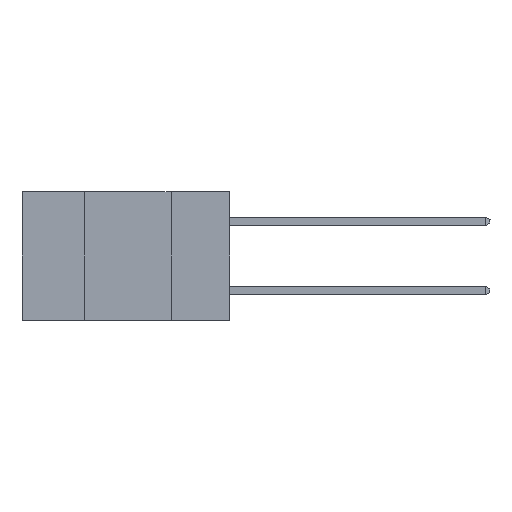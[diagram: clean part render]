
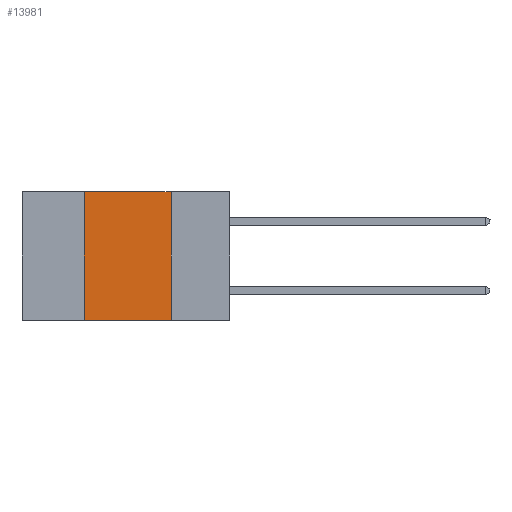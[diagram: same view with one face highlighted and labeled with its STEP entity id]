
A CAD part, left-side view. The second image highlights one B-rep face of the part: STEP entity #13981.
In plain terms, the highlighted planar face has unit normal (-1, 0, 0).
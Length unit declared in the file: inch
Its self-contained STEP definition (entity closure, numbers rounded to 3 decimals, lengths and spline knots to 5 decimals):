
#1023 = DIRECTION ( 'NONE',  ( 0., 0., 1. ) ) ;
#4961 = CARTESIAN_POINT ( 'NONE',  ( 0., 0.6, 0. ) ) ;
#5882 = LINE ( 'NONE', #26419, #10526 ) ;
#6007 = VECTOR ( 'NONE', #11880, 39.37008 ) ;
#7266 = DIRECTION ( 'NONE',  ( 0., 0., -1. ) ) ;
#7350 = FACE_OUTER_BOUND ( 'NONE', #15624, .T. ) ;
#8028 = CARTESIAN_POINT ( 'NONE',  ( 0., 0.42, 0. ) ) ;
#8097 = VECTOR ( 'NONE', #1023, 39.37008 ) ;
#8830 = CARTESIAN_POINT ( 'NONE',  ( 0., 0.42, 0. ) ) ;
#9440 = ORIENTED_EDGE ( 'NONE', *, *, #19440, .F. ) ;
#9848 = PLANE ( 'NONE',  #13588 ) ;
#10526 = VECTOR ( 'NONE', #26039, 39.37008 ) ;
#11048 = LINE ( 'NONE', #26996, #16787 ) ;
#11230 = DIRECTION ( 'NONE',  ( 0., -1., 0. ) ) ;
#11699 = ORIENTED_EDGE ( 'NONE', *, *, #18693, .F. ) ;
#11793 = CARTESIAN_POINT ( 'NONE',  ( 0., 0.6, 0. ) ) ;
#11880 = DIRECTION ( 'NONE',  ( 0., -1., 0. ) ) ;
#13405 = EDGE_CURVE ( 'NONE', #17561, #27401, #5882, .T. ) ;
#13588 = AXIS2_PLACEMENT_3D ( 'NONE', #11793, #23201, #7266 ) ;
#13981 = ADVANCED_FACE ( 'NONE', ( #7350 ), #9848, .F. ) ;
#14949 = LINE ( 'NONE', #8028, #8097 ) ;
#15624 = EDGE_LOOP ( 'NONE', ( #20441, #11699, #9440, #23218 ) ) ;
#16787 = VECTOR ( 'NONE', #11230, 39.37008 ) ;
#17561 = VERTEX_POINT ( 'NONE', #17603 ) ;
#17603 = CARTESIAN_POINT ( 'NONE',  ( 0., 0.17, 0. ) ) ;
#17974 = EDGE_CURVE ( 'NONE', #19180, #27401, #11048, .T. ) ;
#18222 = LINE ( 'NONE', #4961, #6007 ) ;
#18693 = EDGE_CURVE ( 'NONE', #27416, #17561, #18222, .T. ) ;
#19180 = VERTEX_POINT ( 'NONE', #26446 ) ;
#19440 = EDGE_CURVE ( 'NONE', #19180, #27416, #14949, .T. ) ;
#20441 = ORIENTED_EDGE ( 'NONE', *, *, #13405, .F. ) ;
#23201 = DIRECTION ( 'NONE',  ( 1., 0., 0. ) ) ;
#23218 = ORIENTED_EDGE ( 'NONE', *, *, #17974, .T. ) ;
#25037 = CARTESIAN_POINT ( 'NONE',  ( 0., 0.17, -0.37 ) ) ;
#26039 = DIRECTION ( 'NONE',  ( 0., 0., -1. ) ) ;
#26419 = CARTESIAN_POINT ( 'NONE',  ( 0., 0.17, 0. ) ) ;
#26446 = CARTESIAN_POINT ( 'NONE',  ( 0., 0.42, -0.37 ) ) ;
#26996 = CARTESIAN_POINT ( 'NONE',  ( 0., 0.6, -0.37 ) ) ;
#27401 = VERTEX_POINT ( 'NONE', #25037 ) ;
#27416 = VERTEX_POINT ( 'NONE', #8830 ) ;
